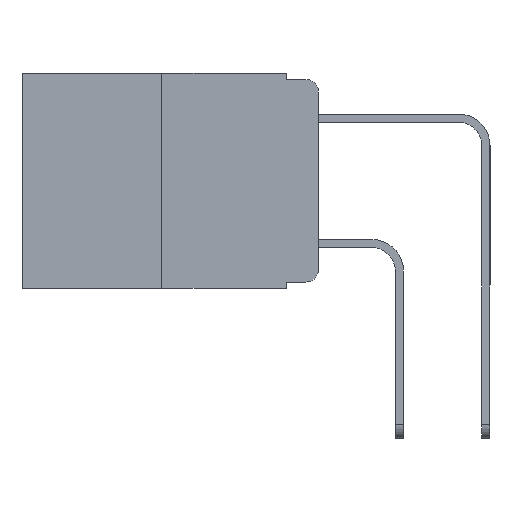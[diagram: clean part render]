
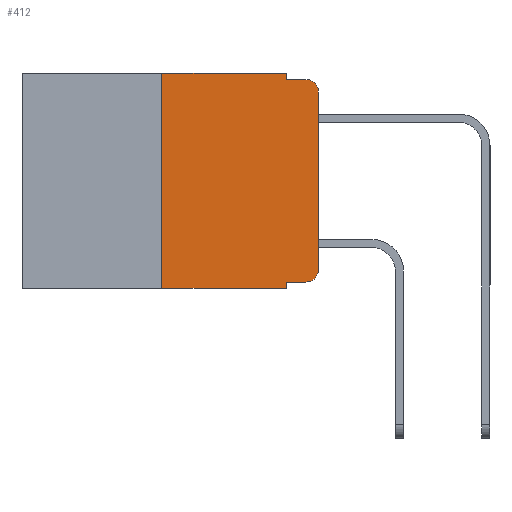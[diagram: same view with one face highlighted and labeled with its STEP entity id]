
A CAD part, left-side view. The second image highlights one B-rep face of the part: STEP entity #412.
In plain terms, the highlighted planar face has unit normal (-1, 0, 0).
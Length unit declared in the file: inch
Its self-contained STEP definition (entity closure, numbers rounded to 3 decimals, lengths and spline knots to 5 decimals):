
#60 = LINE ( 'NONE', #6019, #11615 ) ;
#106 = AXIS2_PLACEMENT_3D ( 'NONE', #2114, #9870, #3282 ) ;
#131 = VERTEX_POINT ( 'NONE', #9655 ) ;
#327 = VERTEX_POINT ( 'NONE', #13229 ) ;
#328 = DIRECTION ( 'NONE',  ( 0., 0., 1. ) ) ;
#344 = VERTEX_POINT ( 'NONE', #837 ) ;
#412 = ADVANCED_FACE ( 'NONE', ( #6181 ), #9355, .F. ) ;
#596 = LINE ( 'NONE', #8177, #6065 ) ;
#837 = CARTESIAN_POINT ( 'NONE',  ( 0., 0.051, -0.01 ) ) ;
#1079 = VECTOR ( 'NONE', #5609, 39.37008 ) ;
#1256 = CIRCLE ( 'NONE', #6002, 0.02 ) ;
#1316 = VERTEX_POINT ( 'NONE', #9610 ) ;
#1395 = EDGE_CURVE ( 'NONE', #12907, #344, #6860, .T. ) ;
#2114 = CARTESIAN_POINT ( 'NONE',  ( 0., 0.02, -0.313 ) ) ;
#2202 = EDGE_CURVE ( 'NONE', #344, #327, #4924, .T. ) ;
#2209 = CARTESIAN_POINT ( 'NONE',  ( 0., 0.051, -0.343 ) ) ;
#2219 = VECTOR ( 'NONE', #3303, 39.37008 ) ;
#2495 = CARTESIAN_POINT ( 'NONE',  ( 0., 0.051, -0.333 ) ) ;
#2570 = CIRCLE ( 'NONE', #106, 0.02 ) ;
#2939 = AXIS2_PLACEMENT_3D ( 'NONE', #11975, #11136, #5262 ) ;
#2979 = EDGE_CURVE ( 'NONE', #131, #327, #1256, .T. ) ;
#3201 = ORIENTED_EDGE ( 'NONE', *, *, #14170, .F. ) ;
#3282 = DIRECTION ( 'NONE',  ( 0., 0., -1. ) ) ;
#3303 = DIRECTION ( 'NONE',  ( 0., -1., 0. ) ) ;
#3551 = EDGE_LOOP ( 'NONE', ( #8930, #13535, #6182, #9286, #7415, #3201, #9298, #8369, #5542, #3857 ) ) ;
#3857 = ORIENTED_EDGE ( 'NONE', *, *, #12019, .T. ) ;
#4333 = VECTOR ( 'NONE', #328, 39.37008 ) ;
#4544 = EDGE_CURVE ( 'NONE', #7254, #131, #8137, .T. ) ;
#4604 = VERTEX_POINT ( 'NONE', #2209 ) ;
#4924 = LINE ( 'NONE', #9438, #2219 ) ;
#5262 = DIRECTION ( 'NONE',  ( 0., 0., -1. ) ) ;
#5542 = ORIENTED_EDGE ( 'NONE', *, *, #12735, .T. ) ;
#5609 = DIRECTION ( 'NONE',  ( 0., -1., 0. ) ) ;
#5805 = VERTEX_POINT ( 'NONE', #2495 ) ;
#5994 = CARTESIAN_POINT ( 'NONE',  ( 0., 0., 0. ) ) ;
#6002 = AXIS2_PLACEMENT_3D ( 'NONE', #7855, #7731, #7683 ) ;
#6019 = CARTESIAN_POINT ( 'NONE',  ( 0., 0.051, 0. ) ) ;
#6065 = VECTOR ( 'NONE', #7075, 39.37008 ) ;
#6181 = FACE_OUTER_BOUND ( 'NONE', #3551, .T. ) ;
#6182 = ORIENTED_EDGE ( 'NONE', *, *, #2202, .F. ) ;
#6183 = DIRECTION ( 'NONE',  ( 0., -1., 0. ) ) ;
#6860 = LINE ( 'NONE', #12884, #11831 ) ;
#7075 = DIRECTION ( 'NONE',  ( 0., -1., 0. ) ) ;
#7128 = DIRECTION ( 'NONE',  ( 0., 0., -1. ) ) ;
#7254 = VERTEX_POINT ( 'NONE', #10547 ) ;
#7281 = LINE ( 'NONE', #11462, #4333 ) ;
#7415 = ORIENTED_EDGE ( 'NONE', *, *, #12388, .F. ) ;
#7480 = DIRECTION ( 'NONE',  ( 0., 0., 1. ) ) ;
#7683 = DIRECTION ( 'NONE',  ( 0., 0., -1. ) ) ;
#7731 = DIRECTION ( 'NONE',  ( -1., 0., 0. ) ) ;
#7855 = CARTESIAN_POINT ( 'NONE',  ( 0., 0.02, -0.03 ) ) ;
#8137 = LINE ( 'NONE', #5994, #10606 ) ;
#8177 = CARTESIAN_POINT ( 'NONE',  ( 0., 0.473, -0.343 ) ) ;
#8369 = ORIENTED_EDGE ( 'NONE', *, *, #13444, .F. ) ;
#8930 = ORIENTED_EDGE ( 'NONE', *, *, #4544, .T. ) ;
#9055 = LINE ( 'NONE', #12586, #11813 ) ;
#9286 = ORIENTED_EDGE ( 'NONE', *, *, #1395, .F. ) ;
#9298 = ORIENTED_EDGE ( 'NONE', *, *, #10091, .T. ) ;
#9355 = PLANE ( 'NONE',  #2939 ) ;
#9438 = CARTESIAN_POINT ( 'NONE',  ( 0., 0.051, -0.01 ) ) ;
#9610 = CARTESIAN_POINT ( 'NONE',  ( 0., 0.02, -0.333 ) ) ;
#9655 = CARTESIAN_POINT ( 'NONE',  ( 0., 0., -0.03 ) ) ;
#9870 = DIRECTION ( 'NONE',  ( -1., 0., 0. ) ) ;
#10091 = EDGE_CURVE ( 'NONE', #11234, #4604, #596, .T. ) ;
#10547 = CARTESIAN_POINT ( 'NONE',  ( 0., 0., -0.313 ) ) ;
#10606 = VECTOR ( 'NONE', #7480, 39.37008 ) ;
#10845 = DIRECTION ( 'NONE',  ( 0., 0., -1. ) ) ;
#11136 = DIRECTION ( 'NONE',  ( 1., 0., 0. ) ) ;
#11234 = VERTEX_POINT ( 'NONE', #13584 ) ;
#11462 = CARTESIAN_POINT ( 'NONE',  ( 0., 0.25, 0. ) ) ;
#11615 = VECTOR ( 'NONE', #7128, 39.37008 ) ;
#11813 = VECTOR ( 'NONE', #6183, 39.37008 ) ;
#11831 = VECTOR ( 'NONE', #10845, 39.37008 ) ;
#11975 = CARTESIAN_POINT ( 'NONE',  ( 0., 0.473, 0. ) ) ;
#12019 = EDGE_CURVE ( 'NONE', #1316, #7254, #2570, .T. ) ;
#12058 = CARTESIAN_POINT ( 'NONE',  ( 0., 0.051, -0.333 ) ) ;
#12388 = EDGE_CURVE ( 'NONE', #12788, #12907, #9055, .T. ) ;
#12481 = LINE ( 'NONE', #12058, #1079 ) ;
#12586 = CARTESIAN_POINT ( 'NONE',  ( 0., 0.473, 0. ) ) ;
#12735 = EDGE_CURVE ( 'NONE', #5805, #1316, #12481, .T. ) ;
#12788 = VERTEX_POINT ( 'NONE', #13225 ) ;
#12884 = CARTESIAN_POINT ( 'NONE',  ( 0., 0.051, 0. ) ) ;
#12907 = VERTEX_POINT ( 'NONE', #13402 ) ;
#13225 = CARTESIAN_POINT ( 'NONE',  ( 0., 0.25, 0. ) ) ;
#13229 = CARTESIAN_POINT ( 'NONE',  ( 0., 0.02, -0.01 ) ) ;
#13402 = CARTESIAN_POINT ( 'NONE',  ( 0., 0.051, 0. ) ) ;
#13444 = EDGE_CURVE ( 'NONE', #5805, #4604, #60, .T. ) ;
#13535 = ORIENTED_EDGE ( 'NONE', *, *, #2979, .T. ) ;
#13584 = CARTESIAN_POINT ( 'NONE',  ( 0., 0.25, -0.343 ) ) ;
#14170 = EDGE_CURVE ( 'NONE', #11234, #12788, #7281, .T. ) ;
